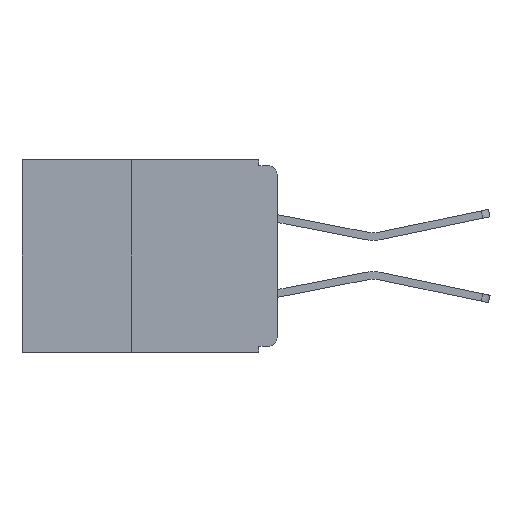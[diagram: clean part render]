
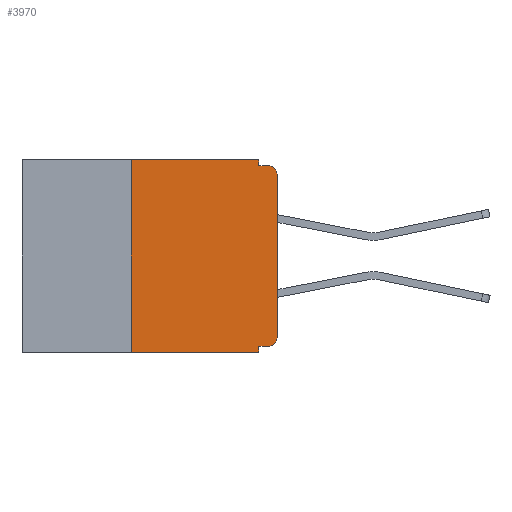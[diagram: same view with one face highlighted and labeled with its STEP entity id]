
A CAD part, left-side view. The second image highlights one B-rep face of the part: STEP entity #3970.
In plain terms, the highlighted planar face has unit normal (-1, 0, 0).
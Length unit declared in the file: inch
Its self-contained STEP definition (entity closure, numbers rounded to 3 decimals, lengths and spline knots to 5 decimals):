
#104 = EDGE_CURVE ( 'NONE', #6326, #2794, #7600, .T. ) ;
#411 = VECTOR ( 'NONE', #2320, 39.37008 ) ;
#672 = VECTOR ( 'NONE', #5782, 39.37008 ) ;
#1338 = VERTEX_POINT ( 'NONE', #7659 ) ;
#1360 = CARTESIAN_POINT ( 'NONE',  ( 0., 0.437, -0.33 ) ) ;
#1395 = EDGE_CURVE ( 'NONE', #6326, #5025, #1846, .T. ) ;
#1513 = ORIENTED_EDGE ( 'NONE', *, *, #7635, .T. ) ;
#1584 = CARTESIAN_POINT ( 'NONE',  ( 0., 0., 0. ) ) ;
#1829 = ORIENTED_EDGE ( 'NONE', *, *, #10781, .F. ) ;
#1844 = VERTEX_POINT ( 'NONE', #11023 ) ;
#1846 = LINE ( 'NONE', #1360, #11005 ) ;
#1860 = DIRECTION ( 'NONE',  ( 0., 0., 1. ) ) ;
#1901 = EDGE_CURVE ( 'NONE', #2794, #4151, #8304, .T. ) ;
#1976 = LINE ( 'NONE', #10813, #11979 ) ;
#2228 = EDGE_CURVE ( 'NONE', #4793, #1844, #12574, .T. ) ;
#2320 = DIRECTION ( 'NONE',  ( 0., -1., 0. ) ) ;
#2436 = CARTESIAN_POINT ( 'NONE',  ( 0., 0.031, 0. ) ) ;
#2669 = EDGE_CURVE ( 'NONE', #7431, #5025, #6371, .T. ) ;
#2716 = CARTESIAN_POINT ( 'NONE',  ( 0., 0.437, 0. ) ) ;
#2774 = ORIENTED_EDGE ( 'NONE', *, *, #7782, .F. ) ;
#2794 = VERTEX_POINT ( 'NONE', #7421 ) ;
#2806 = DIRECTION ( 'NONE',  ( 0., 0., -1. ) ) ;
#2857 = DIRECTION ( 'NONE',  ( -1., 0., 0. ) ) ;
#2873 = DIRECTION ( 'NONE',  ( 0., -1., 0. ) ) ;
#3427 = LINE ( 'NONE', #4741, #672 ) ;
#3739 = VECTOR ( 'NONE', #11479, 39.37008 ) ;
#3899 = ORIENTED_EDGE ( 'NONE', *, *, #7181, .T. ) ;
#3970 = ADVANCED_FACE ( 'NONE', ( #9888 ), #11804, .F. ) ;
#3972 = AXIS2_PLACEMENT_3D ( 'NONE', #8706, #2857, #9700 ) ;
#4151 = VERTEX_POINT ( 'NONE', #2436 ) ;
#4168 = CIRCLE ( 'NONE', #3972, 0.015 ) ;
#4182 = CARTESIAN_POINT ( 'NONE',  ( 0., 0.437, 0. ) ) ;
#4441 = VERTEX_POINT ( 'NONE', #11982 ) ;
#4515 = CARTESIAN_POINT ( 'NONE',  ( 0., 0.25, -0.33 ) ) ;
#4741 = CARTESIAN_POINT ( 'NONE',  ( 0., 0.031, 0. ) ) ;
#4745 = CARTESIAN_POINT ( 'NONE',  ( 0., 0.031, -0.33 ) ) ;
#4793 = VERTEX_POINT ( 'NONE', #5666 ) ;
#5025 = VERTEX_POINT ( 'NONE', #6036 ) ;
#5107 = ORIENTED_EDGE ( 'NONE', *, *, #2669, .F. ) ;
#5437 = ORIENTED_EDGE ( 'NONE', *, *, #5760, .T. ) ;
#5666 = CARTESIAN_POINT ( 'NONE',  ( 0., 0.031, -0.01 ) ) ;
#5760 = EDGE_CURVE ( 'NONE', #9162, #4441, #5795, .T. ) ;
#5782 = DIRECTION ( 'NONE',  ( 0., 0., -1. ) ) ;
#5795 = CIRCLE ( 'NONE', #6999, 0.015 ) ;
#6020 = EDGE_LOOP ( 'NONE', ( #3899, #1513, #6831, #1829, #7108, #12132, #7415, #5107, #2774, #5437 ) ) ;
#6036 = CARTESIAN_POINT ( 'NONE',  ( 0., 0.031, -0.33 ) ) ;
#6326 = VERTEX_POINT ( 'NONE', #4515 ) ;
#6371 = LINE ( 'NONE', #4745, #3739 ) ;
#6831 = ORIENTED_EDGE ( 'NONE', *, *, #2228, .F. ) ;
#6999 = AXIS2_PLACEMENT_3D ( 'NONE', #12096, #12044, #11317 ) ;
#7108 = ORIENTED_EDGE ( 'NONE', *, *, #1901, .F. ) ;
#7181 = EDGE_CURVE ( 'NONE', #4441, #1338, #9066, .T. ) ;
#7415 = ORIENTED_EDGE ( 'NONE', *, *, #1395, .T. ) ;
#7421 = CARTESIAN_POINT ( 'NONE',  ( 0., 0.25, 0. ) ) ;
#7431 = VERTEX_POINT ( 'NONE', #11259 ) ;
#7600 = LINE ( 'NONE', #11001, #9865 ) ;
#7635 = EDGE_CURVE ( 'NONE', #1338, #1844, #4168, .T. ) ;
#7659 = CARTESIAN_POINT ( 'NONE',  ( 0., 0., -0.025 ) ) ;
#7782 = EDGE_CURVE ( 'NONE', #9162, #7431, #1976, .T. ) ;
#8304 = LINE ( 'NONE', #4182, #411 ) ;
#8706 = CARTESIAN_POINT ( 'NONE',  ( 0., 0.015, -0.025 ) ) ;
#8737 = DIRECTION ( 'NONE',  ( 1., 0., 0. ) ) ;
#8934 = DIRECTION ( 'NONE',  ( 0., 1., 0. ) ) ;
#9066 = LINE ( 'NONE', #1584, #11571 ) ;
#9162 = VERTEX_POINT ( 'NONE', #10123 ) ;
#9533 = VECTOR ( 'NONE', #10132, 39.37008 ) ;
#9700 = DIRECTION ( 'NONE',  ( 0., 0., -1. ) ) ;
#9865 = VECTOR ( 'NONE', #11067, 39.37008 ) ;
#9888 = FACE_OUTER_BOUND ( 'NONE', #6020, .T. ) ;
#9915 = AXIS2_PLACEMENT_3D ( 'NONE', #2716, #8737, #2806 ) ;
#10123 = CARTESIAN_POINT ( 'NONE',  ( 0., 0.015, -0.32 ) ) ;
#10132 = DIRECTION ( 'NONE',  ( 0., -1., 0. ) ) ;
#10172 = CARTESIAN_POINT ( 'NONE',  ( 0., 0., -0.01 ) ) ;
#10781 = EDGE_CURVE ( 'NONE', #4151, #4793, #3427, .T. ) ;
#10813 = CARTESIAN_POINT ( 'NONE',  ( 0., 0., -0.32 ) ) ;
#11001 = CARTESIAN_POINT ( 'NONE',  ( 0., 0.25, -0.33 ) ) ;
#11005 = VECTOR ( 'NONE', #2873, 39.37008 ) ;
#11023 = CARTESIAN_POINT ( 'NONE',  ( 0., 0.015, -0.01 ) ) ;
#11067 = DIRECTION ( 'NONE',  ( 0., 0., 1. ) ) ;
#11259 = CARTESIAN_POINT ( 'NONE',  ( 0., 0.031, -0.32 ) ) ;
#11317 = DIRECTION ( 'NONE',  ( 0., 0., -1. ) ) ;
#11479 = DIRECTION ( 'NONE',  ( 0., 0., -1. ) ) ;
#11571 = VECTOR ( 'NONE', #1860, 39.37008 ) ;
#11804 = PLANE ( 'NONE',  #9915 ) ;
#11979 = VECTOR ( 'NONE', #8934, 39.37008 ) ;
#11982 = CARTESIAN_POINT ( 'NONE',  ( 0., 0., -0.305 ) ) ;
#12044 = DIRECTION ( 'NONE',  ( -1., 0., 0. ) ) ;
#12096 = CARTESIAN_POINT ( 'NONE',  ( 0., 0.015, -0.305 ) ) ;
#12132 = ORIENTED_EDGE ( 'NONE', *, *, #104, .F. ) ;
#12574 = LINE ( 'NONE', #10172, #9533 ) ;
